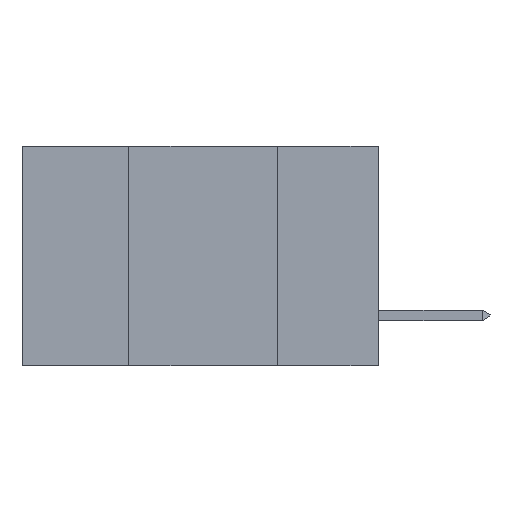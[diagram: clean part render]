
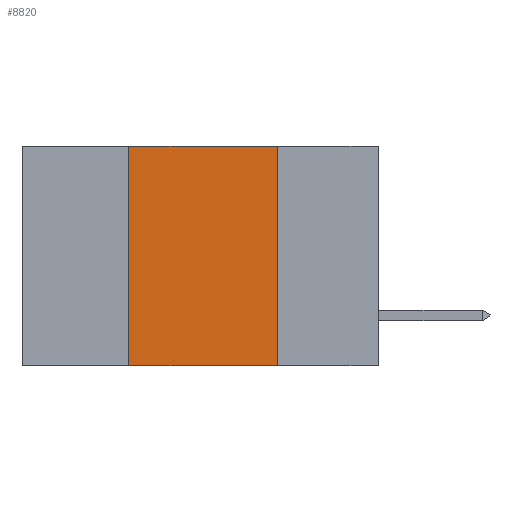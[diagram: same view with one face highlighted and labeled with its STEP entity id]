
A CAD part, left-side view. The second image highlights one B-rep face of the part: STEP entity #8820.
In plain terms, the highlighted planar face has unit normal (-1, 0, 0).
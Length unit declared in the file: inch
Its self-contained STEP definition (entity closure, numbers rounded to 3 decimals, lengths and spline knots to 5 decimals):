
#388 = VECTOR ( 'NONE', #13287, 39.37008 ) ;
#1548 = CARTESIAN_POINT ( 'NONE',  ( 0., 0.6, 0. ) ) ;
#1834 = EDGE_CURVE ( 'NONE', #4602, #14529, #11669, .T. ) ;
#2201 = LINE ( 'NONE', #9198, #388 ) ;
#4557 = EDGE_CURVE ( 'NONE', #6797, #14529, #6266, .T. ) ;
#4602 = VERTEX_POINT ( 'NONE', #7619 ) ;
#5867 = DIRECTION ( 'NONE',  ( 0., 0., -1. ) ) ;
#6266 = LINE ( 'NONE', #10322, #12278 ) ;
#6797 = VERTEX_POINT ( 'NONE', #14715 ) ;
#7116 = ORIENTED_EDGE ( 'NONE', *, *, #4557, .F. ) ;
#7376 = CARTESIAN_POINT ( 'NONE',  ( 0., 0.17, -0.37 ) ) ;
#7447 = EDGE_CURVE ( 'NONE', #10998, #6797, #2201, .T. ) ;
#7619 = CARTESIAN_POINT ( 'NONE',  ( 0., 0.42, -0.37 ) ) ;
#7755 = EDGE_LOOP ( 'NONE', ( #7116, #16583, #11687, #11673 ) ) ;
#7792 = VECTOR ( 'NONE', #10306, 39.37008 ) ;
#8820 = ADVANCED_FACE ( 'NONE', ( #14099 ), #17068, .F. ) ;
#9198 = CARTESIAN_POINT ( 'NONE',  ( 0., 0.6, 0. ) ) ;
#9600 = CARTESIAN_POINT ( 'NONE',  ( 0., 0.42, 0. ) ) ;
#9825 = EDGE_CURVE ( 'NONE', #4602, #10998, #11416, .T. ) ;
#10306 = DIRECTION ( 'NONE',  ( 0., -1., 0. ) ) ;
#10322 = CARTESIAN_POINT ( 'NONE',  ( 0., 0.17, -0.37 ) ) ;
#10998 = VERTEX_POINT ( 'NONE', #9600 ) ;
#11416 = LINE ( 'NONE', #13959, #14386 ) ;
#11669 = LINE ( 'NONE', #17192, #7792 ) ;
#11673 = ORIENTED_EDGE ( 'NONE', *, *, #1834, .T. ) ;
#11687 = ORIENTED_EDGE ( 'NONE', *, *, #9825, .F. ) ;
#11855 = DIRECTION ( 'NONE',  ( 0., 0., -1. ) ) ;
#12278 = VECTOR ( 'NONE', #11855, 39.37008 ) ;
#13287 = DIRECTION ( 'NONE',  ( 0., -1., 0. ) ) ;
#13800 = AXIS2_PLACEMENT_3D ( 'NONE', #1548, #14271, #5867 ) ;
#13878 = DIRECTION ( 'NONE',  ( 0., 0., 1. ) ) ;
#13959 = CARTESIAN_POINT ( 'NONE',  ( 0., 0.42, -0.37 ) ) ;
#14099 = FACE_OUTER_BOUND ( 'NONE', #7755, .T. ) ;
#14271 = DIRECTION ( 'NONE',  ( 1., 0., 0. ) ) ;
#14386 = VECTOR ( 'NONE', #13878, 39.37008 ) ;
#14529 = VERTEX_POINT ( 'NONE', #7376 ) ;
#14715 = CARTESIAN_POINT ( 'NONE',  ( 0., 0.17, 0. ) ) ;
#16583 = ORIENTED_EDGE ( 'NONE', *, *, #7447, .F. ) ;
#17068 = PLANE ( 'NONE',  #13800 ) ;
#17192 = CARTESIAN_POINT ( 'NONE',  ( 0., 0.6, -0.37 ) ) ;
